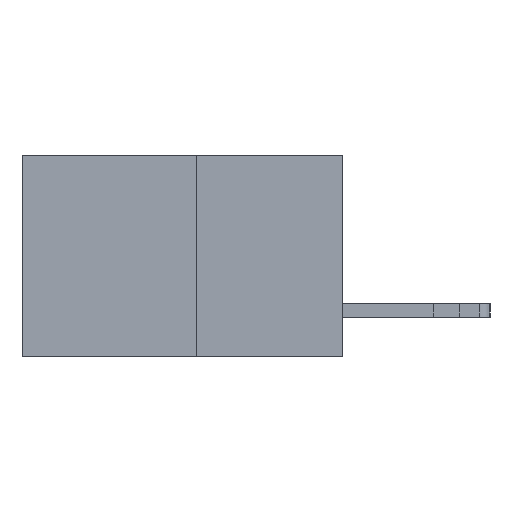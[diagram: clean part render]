
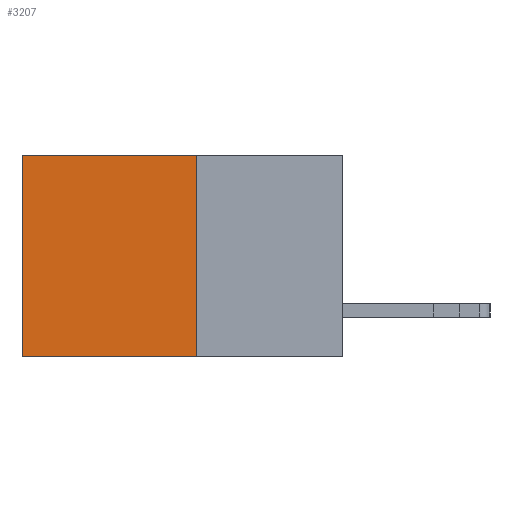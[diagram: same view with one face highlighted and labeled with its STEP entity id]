
A CAD part, left-side view. The second image highlights one B-rep face of the part: STEP entity #3207.
In plain terms, the highlighted planar face has unit normal (-1, 0, 0).
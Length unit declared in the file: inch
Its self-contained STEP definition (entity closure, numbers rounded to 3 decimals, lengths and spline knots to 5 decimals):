
#1359 = LINE ( 'NONE', #20009, #22640 ) ;
#1444 = CARTESIAN_POINT ( 'NONE',  ( 0.277, 0.27, -0.37 ) ) ;
#1718 = DIRECTION ( 'NONE',  ( 1., 0., 0. ) ) ;
#2045 = VERTEX_POINT ( 'NONE', #9154 ) ;
#3207 = ADVANCED_FACE ( 'NONE', ( #18596 ), #13392, .F. ) ;
#3274 = LINE ( 'NONE', #19778, #19196 ) ;
#5709 = EDGE_CURVE ( 'NONE', #14952, #2045, #18128, .T. ) ;
#6383 = LINE ( 'NONE', #17155, #21542 ) ;
#7468 = EDGE_CURVE ( 'NONE', #25480, #7726, #6383, .T. ) ;
#7726 = VERTEX_POINT ( 'NONE', #1444 ) ;
#9154 = CARTESIAN_POINT ( 'NONE',  ( 0.277, 0.59, -0.37 ) ) ;
#9956 = DIRECTION ( 'NONE',  ( 0., 0., -1. ) ) ;
#10381 = CARTESIAN_POINT ( 'NONE',  ( 0.277, 0.59, -0.37 ) ) ;
#11060 = CARTESIAN_POINT ( 'NONE',  ( 0.277, 0.27, -0.37 ) ) ;
#11318 = DIRECTION ( 'NONE',  ( 0., 0., -1. ) ) ;
#11801 = DIRECTION ( 'NONE',  ( 0., 1., 0. ) ) ;
#11990 = VECTOR ( 'NONE', #9956, 39.37008 ) ;
#13392 = PLANE ( 'NONE',  #15000 ) ;
#14215 = ORIENTED_EDGE ( 'NONE', *, *, #18830, .F. ) ;
#14598 = EDGE_LOOP ( 'NONE', ( #21904, #14215, #20413, #18469 ) ) ;
#14952 = VERTEX_POINT ( 'NONE', #20566 ) ;
#15000 = AXIS2_PLACEMENT_3D ( 'NONE', #11060, #1718, #11318 ) ;
#15145 = DIRECTION ( 'NONE',  ( 0., 0., -1. ) ) ;
#17155 = CARTESIAN_POINT ( 'NONE',  ( 0.277, 0.27, -0.37 ) ) ;
#18128 = LINE ( 'NONE', #10381, #11990 ) ;
#18469 = ORIENTED_EDGE ( 'NONE', *, *, #19630, .T. ) ;
#18596 = FACE_OUTER_BOUND ( 'NONE', #14598, .T. ) ;
#18830 = EDGE_CURVE ( 'NONE', #7726, #2045, #3274, .T. ) ;
#19196 = VECTOR ( 'NONE', #21789, 39.37008 ) ;
#19630 = EDGE_CURVE ( 'NONE', #25480, #14952, #1359, .T. ) ;
#19778 = CARTESIAN_POINT ( 'NONE',  ( 0.277, 0.27, -0.37 ) ) ;
#20009 = CARTESIAN_POINT ( 'NONE',  ( 0.277, 0.27, 0. ) ) ;
#20413 = ORIENTED_EDGE ( 'NONE', *, *, #7468, .F. ) ;
#20566 = CARTESIAN_POINT ( 'NONE',  ( 0.277, 0.59, 0. ) ) ;
#21542 = VECTOR ( 'NONE', #15145, 39.37008 ) ;
#21789 = DIRECTION ( 'NONE',  ( 0., 1., 0. ) ) ;
#21904 = ORIENTED_EDGE ( 'NONE', *, *, #5709, .T. ) ;
#22640 = VECTOR ( 'NONE', #11801, 39.37008 ) ;
#24772 = CARTESIAN_POINT ( 'NONE',  ( 0.277, 0.27, 0. ) ) ;
#25480 = VERTEX_POINT ( 'NONE', #24772 ) ;
